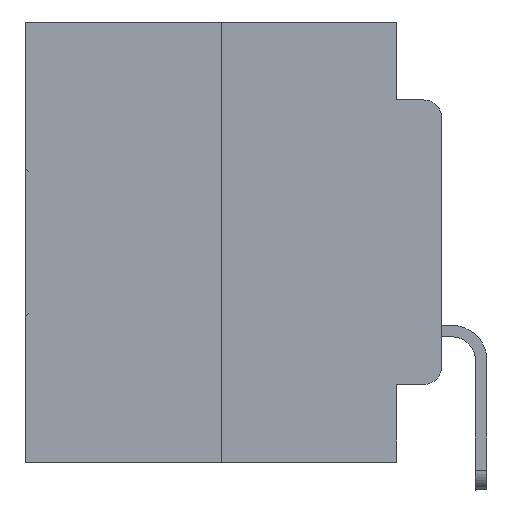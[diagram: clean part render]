
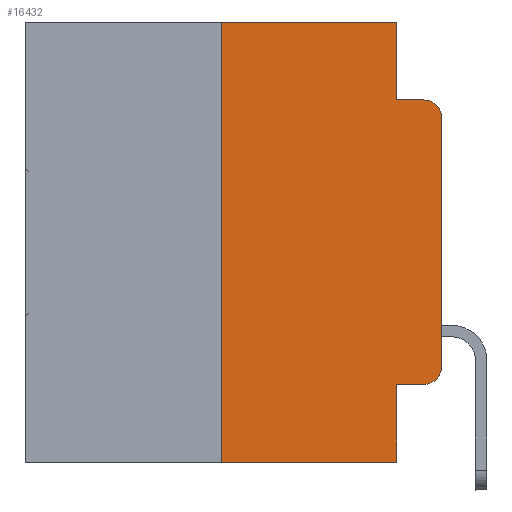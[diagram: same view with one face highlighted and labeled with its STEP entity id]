
A CAD part, left-side view. The second image highlights one B-rep face of the part: STEP entity #16432.
In plain terms, the highlighted planar face has unit normal (-1, 0, 0).
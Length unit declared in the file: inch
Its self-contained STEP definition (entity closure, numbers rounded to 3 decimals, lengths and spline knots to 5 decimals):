
#99 = CARTESIAN_POINT ( 'NONE',  ( 0., 0.051, 0. ) ) ;
#162 = CARTESIAN_POINT ( 'NONE',  ( 0., 0.051, -0.0885 ) ) ;
#252 = VERTEX_POINT ( 'NONE', #13031 ) ;
#380 = VECTOR ( 'NONE', #4952, 39.37008 ) ;
#589 = ORIENTED_EDGE ( 'NONE', *, *, #28402, .T. ) ;
#1470 = DIRECTION ( 'NONE',  ( 0., 0., 1. ) ) ;
#1600 = VERTEX_POINT ( 'NONE', #13182 ) ;
#2176 = AXIS2_PLACEMENT_3D ( 'NONE', #11644, #18779, #21135 ) ;
#2298 = EDGE_CURVE ( 'NONE', #21164, #23484, #2860, .T. ) ;
#2860 = LINE ( 'NONE', #99, #12416 ) ;
#3377 = CARTESIAN_POINT ( 'NONE',  ( 0., 0.25, -0.5 ) ) ;
#3386 = DIRECTION ( 'NONE',  ( 0., 0., -1. ) ) ;
#3716 = CIRCLE ( 'NONE', #30016, 0.02 ) ;
#3786 = EDGE_LOOP ( 'NONE', ( #24732, #23341, #5778, #29934, #24534, #28361, #26240, #16574, #18973, #589 ) ) ;
#3793 = LINE ( 'NONE', #11240, #15044 ) ;
#3796 = EDGE_CURVE ( 'NONE', #18418, #17333, #25162, .T. ) ;
#4124 = VERTEX_POINT ( 'NONE', #21844 ) ;
#4642 = FACE_OUTER_BOUND ( 'NONE', #3786, .T. ) ;
#4815 = LINE ( 'NONE', #162, #13419 ) ;
#4952 = DIRECTION ( 'NONE',  ( 0., -1., 0. ) ) ;
#5343 = EDGE_CURVE ( 'NONE', #13340, #252, #15809, .T. ) ;
#5647 = VECTOR ( 'NONE', #28267, 39.37008 ) ;
#5778 = ORIENTED_EDGE ( 'NONE', *, *, #14325, .F. ) ;
#6497 = DIRECTION ( 'NONE',  ( -1., 0., 0. ) ) ;
#6647 = EDGE_CURVE ( 'NONE', #21794, #1600, #3716, .T. ) ;
#7394 = VECTOR ( 'NONE', #14516, 39.37008 ) ;
#7583 = VECTOR ( 'NONE', #3386, 39.37008 ) ;
#7957 = CARTESIAN_POINT ( 'NONE',  ( 0., 0.051, -0.5 ) ) ;
#8036 = CARTESIAN_POINT ( 'NONE',  ( 0., 0.02, -0.4115 ) ) ;
#9457 = VECTOR ( 'NONE', #1470, 39.37008 ) ;
#9687 = CARTESIAN_POINT ( 'NONE',  ( 0., 0.051, -0.4115 ) ) ;
#9830 = LINE ( 'NONE', #9687, #7394 ) ;
#10634 = CARTESIAN_POINT ( 'NONE',  ( 0., 0.051, -0.4115 ) ) ;
#11083 = DIRECTION ( 'NONE',  ( 0., -1., 0. ) ) ;
#11240 = CARTESIAN_POINT ( 'NONE',  ( 0., 0.473, -0.5 ) ) ;
#11644 = CARTESIAN_POINT ( 'NONE',  ( 0., 0.473, 0. ) ) ;
#12171 = EDGE_CURVE ( 'NONE', #18418, #18405, #9830, .T. ) ;
#12416 = VECTOR ( 'NONE', #23895, 39.37008 ) ;
#12998 = LINE ( 'NONE', #27141, #9457 ) ;
#13031 = CARTESIAN_POINT ( 'NONE',  ( 0., 0.25, 0. ) ) ;
#13182 = CARTESIAN_POINT ( 'NONE',  ( 0., 0.02, -0.0885 ) ) ;
#13340 = VERTEX_POINT ( 'NONE', #3377 ) ;
#13419 = VECTOR ( 'NONE', #21608, 39.37008 ) ;
#13736 = EDGE_CURVE ( 'NONE', #4124, #21794, #12998, .T. ) ;
#14325 = EDGE_CURVE ( 'NONE', #23484, #1600, #4815, .T. ) ;
#14516 = DIRECTION ( 'NONE',  ( 0., -1., 0. ) ) ;
#15044 = VECTOR ( 'NONE', #11083, 39.37008 ) ;
#15226 = CARTESIAN_POINT ( 'NONE',  ( 0., 0.051, 0. ) ) ;
#15809 = LINE ( 'NONE', #16270, #5647 ) ;
#16098 = CARTESIAN_POINT ( 'NONE',  ( 0., 0., -0.1085 ) ) ;
#16270 = CARTESIAN_POINT ( 'NONE',  ( 0., 0.25, 0. ) ) ;
#16432 = ADVANCED_FACE ( 'NONE', ( #4642 ), #21296, .F. ) ;
#16453 = DIRECTION ( 'NONE',  ( -1., 0., 0. ) ) ;
#16574 = ORIENTED_EDGE ( 'NONE', *, *, #3796, .F. ) ;
#16759 = LINE ( 'NONE', #21453, #380 ) ;
#17333 = VERTEX_POINT ( 'NONE', #7957 ) ;
#18405 = VERTEX_POINT ( 'NONE', #8036 ) ;
#18418 = VERTEX_POINT ( 'NONE', #10634 ) ;
#18779 = DIRECTION ( 'NONE',  ( 1., 0., 0. ) ) ;
#18921 = CARTESIAN_POINT ( 'NONE',  ( 0., 0.02, -0.1085 ) ) ;
#18973 = ORIENTED_EDGE ( 'NONE', *, *, #12171, .T. ) ;
#19880 = CARTESIAN_POINT ( 'NONE',  ( 0., 0.051, 0. ) ) ;
#21135 = DIRECTION ( 'NONE',  ( 0., 0., -1. ) ) ;
#21164 = VERTEX_POINT ( 'NONE', #15226 ) ;
#21294 = DIRECTION ( 'NONE',  ( 0., 0., -1. ) ) ;
#21296 = PLANE ( 'NONE',  #2176 ) ;
#21453 = CARTESIAN_POINT ( 'NONE',  ( 0., 0.473, 0. ) ) ;
#21608 = DIRECTION ( 'NONE',  ( 0., -1., 0. ) ) ;
#21742 = CIRCLE ( 'NONE', #28682, 0.02 ) ;
#21794 = VERTEX_POINT ( 'NONE', #16098 ) ;
#21844 = CARTESIAN_POINT ( 'NONE',  ( 0., 0., -0.3915 ) ) ;
#23341 = ORIENTED_EDGE ( 'NONE', *, *, #6647, .T. ) ;
#23484 = VERTEX_POINT ( 'NONE', #25374 ) ;
#23895 = DIRECTION ( 'NONE',  ( 0., 0., -1. ) ) ;
#24534 = ORIENTED_EDGE ( 'NONE', *, *, #28557, .F. ) ;
#24732 = ORIENTED_EDGE ( 'NONE', *, *, #13736, .T. ) ;
#25162 = LINE ( 'NONE', #19880, #7583 ) ;
#25374 = CARTESIAN_POINT ( 'NONE',  ( 0., 0.051, -0.0885 ) ) ;
#26240 = ORIENTED_EDGE ( 'NONE', *, *, #27891, .T. ) ;
#27141 = CARTESIAN_POINT ( 'NONE',  ( 0., 0., 0. ) ) ;
#27891 = EDGE_CURVE ( 'NONE', #13340, #17333, #3793, .T. ) ;
#28267 = DIRECTION ( 'NONE',  ( 0., 0., 1. ) ) ;
#28272 = DIRECTION ( 'NONE',  ( 0., 0., -1. ) ) ;
#28290 = CARTESIAN_POINT ( 'NONE',  ( 0., 0.02, -0.3915 ) ) ;
#28361 = ORIENTED_EDGE ( 'NONE', *, *, #5343, .F. ) ;
#28402 = EDGE_CURVE ( 'NONE', #18405, #4124, #21742, .T. ) ;
#28557 = EDGE_CURVE ( 'NONE', #252, #21164, #16759, .T. ) ;
#28682 = AXIS2_PLACEMENT_3D ( 'NONE', #28290, #16453, #21294 ) ;
#29934 = ORIENTED_EDGE ( 'NONE', *, *, #2298, .F. ) ;
#30016 = AXIS2_PLACEMENT_3D ( 'NONE', #18921, #6497, #28272 ) ;
